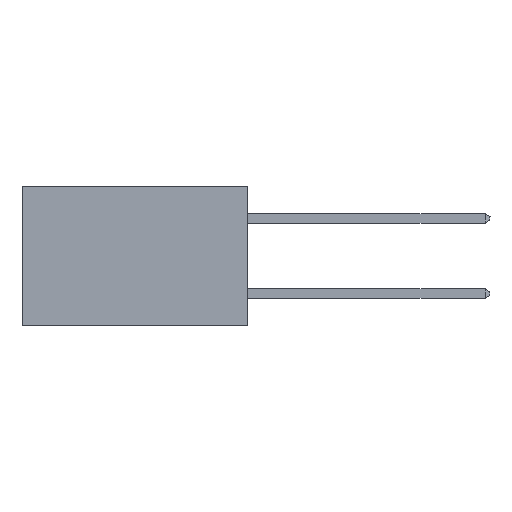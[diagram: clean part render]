
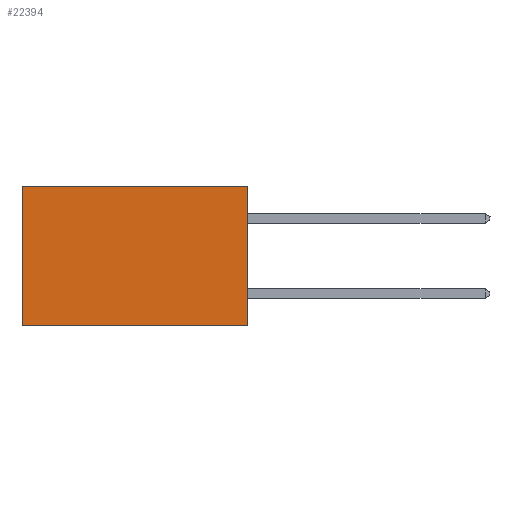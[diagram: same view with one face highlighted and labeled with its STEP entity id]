
A CAD part, left-side view. The second image highlights one B-rep face of the part: STEP entity #22394.
In plain terms, the highlighted planar face has unit normal (-1, 0, 0).
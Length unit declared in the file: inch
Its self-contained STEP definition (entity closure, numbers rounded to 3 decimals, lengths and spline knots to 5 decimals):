
#513 = ORIENTED_EDGE ( 'NONE', *, *, #11448, .F. ) ;
#585 = PLANE ( 'NONE',  #694 ) ;
#694 = AXIS2_PLACEMENT_3D ( 'NONE', #11161, #21736, #11281 ) ;
#1434 = LINE ( 'NONE', #5403, #20953 ) ;
#1610 = ORIENTED_EDGE ( 'NONE', *, *, #8782, .T. ) ;
#1647 = CARTESIAN_POINT ( 'NONE',  ( 0.2615, 0., 0. ) ) ;
#2688 = CARTESIAN_POINT ( 'NONE',  ( 0.2615, 0.6, 0. ) ) ;
#2702 = CARTESIAN_POINT ( 'NONE',  ( 0.2615, 0., -0.37 ) ) ;
#2956 = VECTOR ( 'NONE', #20558, 39.37008 ) ;
#4460 = CARTESIAN_POINT ( 'NONE',  ( 0.2615, 0., -0.37 ) ) ;
#5212 = DIRECTION ( 'NONE',  ( 0., 0., -1. ) ) ;
#5403 = CARTESIAN_POINT ( 'NONE',  ( 0.2615, 0., -0.37 ) ) ;
#7403 = ORIENTED_EDGE ( 'NONE', *, *, #22352, .F. ) ;
#7860 = FACE_OUTER_BOUND ( 'NONE', #12593, .T. ) ;
#8361 = VERTEX_POINT ( 'NONE', #2702 ) ;
#8587 = DIRECTION ( 'NONE',  ( 0., 1., 0. ) ) ;
#8782 = EDGE_CURVE ( 'NONE', #18250, #13799, #9948, .T. ) ;
#9948 = LINE ( 'NONE', #11962, #22355 ) ;
#10392 = ORIENTED_EDGE ( 'NONE', *, *, #10651, .T. ) ;
#10651 = EDGE_CURVE ( 'NONE', #13799, #18367, #15808, .T. ) ;
#10743 = CARTESIAN_POINT ( 'NONE',  ( 0.2615, 0.6, -0.37 ) ) ;
#11161 = CARTESIAN_POINT ( 'NONE',  ( 0.2615, 0., -0.37 ) ) ;
#11281 = DIRECTION ( 'NONE',  ( 0., 0., -1. ) ) ;
#11448 = EDGE_CURVE ( 'NONE', #18250, #8361, #13177, .T. ) ;
#11727 = DIRECTION ( 'NONE',  ( 0., 1., 0. ) ) ;
#11962 = CARTESIAN_POINT ( 'NONE',  ( 0.2615, 0., 0. ) ) ;
#12347 = CARTESIAN_POINT ( 'NONE',  ( 0.2615, 0.6, -0.37 ) ) ;
#12593 = EDGE_LOOP ( 'NONE', ( #10392, #7403, #513, #1610 ) ) ;
#13177 = LINE ( 'NONE', #4460, #2956 ) ;
#13799 = VERTEX_POINT ( 'NONE', #2688 ) ;
#14539 = VECTOR ( 'NONE', #5212, 39.37008 ) ;
#15808 = LINE ( 'NONE', #10743, #14539 ) ;
#18250 = VERTEX_POINT ( 'NONE', #1647 ) ;
#18367 = VERTEX_POINT ( 'NONE', #12347 ) ;
#20558 = DIRECTION ( 'NONE',  ( 0., 0., -1. ) ) ;
#20953 = VECTOR ( 'NONE', #8587, 39.37008 ) ;
#21736 = DIRECTION ( 'NONE',  ( 1., 0., 0. ) ) ;
#22352 = EDGE_CURVE ( 'NONE', #8361, #18367, #1434, .T. ) ;
#22355 = VECTOR ( 'NONE', #11727, 39.37008 ) ;
#22394 = ADVANCED_FACE ( 'NONE', ( #7860 ), #585, .F. ) ;
